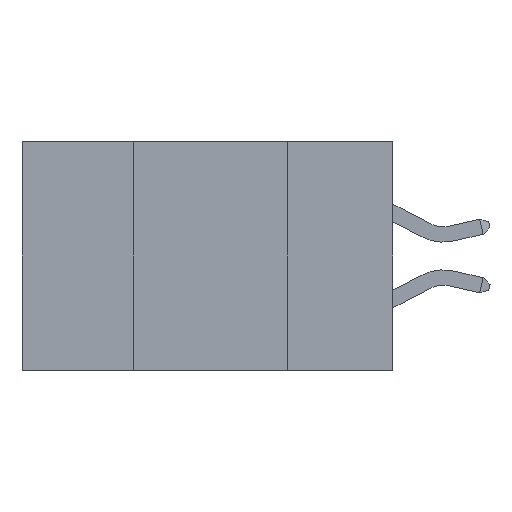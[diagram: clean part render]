
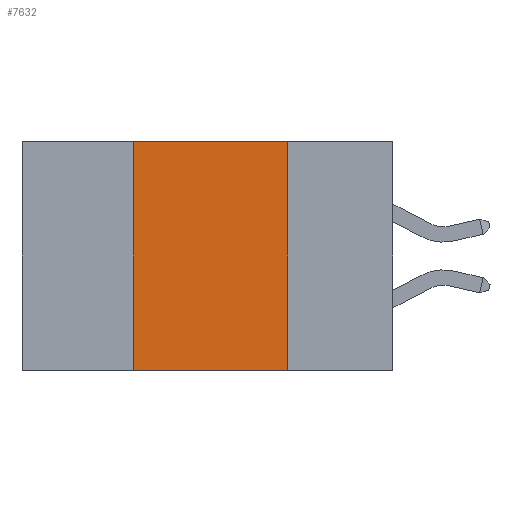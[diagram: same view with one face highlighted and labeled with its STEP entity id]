
A CAD part, left-side view. The second image highlights one B-rep face of the part: STEP entity #7632.
In plain terms, the highlighted planar face has unit normal (-1, 0, 0).
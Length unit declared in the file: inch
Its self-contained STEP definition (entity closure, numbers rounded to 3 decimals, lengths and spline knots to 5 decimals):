
#24 = EDGE_CURVE ( 'NONE', #8611, #7812, #4226, .T. ) ;
#642 = DIRECTION ( 'NONE',  ( 1., 0., 0. ) ) ;
#860 = DIRECTION ( 'NONE',  ( 0., -1., 0. ) ) ;
#1058 = ORIENTED_EDGE ( 'NONE', *, *, #3989, .F. ) ;
#1064 = ORIENTED_EDGE ( 'NONE', *, *, #24, .F. ) ;
#1404 = PLANE ( 'NONE',  #4355 ) ;
#1653 = CARTESIAN_POINT ( 'NONE',  ( 0., 0.17, 0. ) ) ;
#1796 = LINE ( 'NONE', #3952, #2019 ) ;
#1858 = LINE ( 'NONE', #4236, #2079 ) ;
#2019 = VECTOR ( 'NONE', #2530, 39.37008 ) ;
#2022 = DIRECTION ( 'NONE',  ( 0., 0., -1. ) ) ;
#2079 = VECTOR ( 'NONE', #2022, 39.37008 ) ;
#2214 = VECTOR ( 'NONE', #5422, 39.37008 ) ;
#2347 = CARTESIAN_POINT ( 'NONE',  ( 0., 0.6, -0.37 ) ) ;
#2530 = DIRECTION ( 'NONE',  ( 0., -1., 0. ) ) ;
#3100 = FACE_OUTER_BOUND ( 'NONE', #8077, .T. ) ;
#3587 = VERTEX_POINT ( 'NONE', #8003 ) ;
#3935 = EDGE_CURVE ( 'NONE', #8611, #3587, #5152, .T. ) ;
#3952 = CARTESIAN_POINT ( 'NONE',  ( 0., 0.6, 0. ) ) ;
#3989 = EDGE_CURVE ( 'NONE', #7812, #6988, #1796, .T. ) ;
#4226 = LINE ( 'NONE', #8177, #2214 ) ;
#4236 = CARTESIAN_POINT ( 'NONE',  ( 0., 0.17, 0. ) ) ;
#4355 = AXIS2_PLACEMENT_3D ( 'NONE', #8483, #642, #5683 ) ;
#5152 = LINE ( 'NONE', #2347, #7651 ) ;
#5422 = DIRECTION ( 'NONE',  ( 0., 0., 1. ) ) ;
#5683 = DIRECTION ( 'NONE',  ( 0., 0., -1. ) ) ;
#6988 = VERTEX_POINT ( 'NONE', #1653 ) ;
#7632 = ADVANCED_FACE ( 'NONE', ( #3100 ), #1404, .F. ) ;
#7651 = VECTOR ( 'NONE', #860, 39.37008 ) ;
#7812 = VERTEX_POINT ( 'NONE', #7968 ) ;
#7908 = ORIENTED_EDGE ( 'NONE', *, *, #7946, .F. ) ;
#7946 = EDGE_CURVE ( 'NONE', #6988, #3587, #1858, .T. ) ;
#7965 = CARTESIAN_POINT ( 'NONE',  ( 0., 0.42, -0.37 ) ) ;
#7968 = CARTESIAN_POINT ( 'NONE',  ( 0., 0.42, 0. ) ) ;
#8003 = CARTESIAN_POINT ( 'NONE',  ( 0., 0.17, -0.37 ) ) ;
#8077 = EDGE_LOOP ( 'NONE', ( #7908, #1058, #1064, #8278 ) ) ;
#8177 = CARTESIAN_POINT ( 'NONE',  ( 0., 0.42, 0. ) ) ;
#8278 = ORIENTED_EDGE ( 'NONE', *, *, #3935, .T. ) ;
#8483 = CARTESIAN_POINT ( 'NONE',  ( 0., 0.6, 0. ) ) ;
#8611 = VERTEX_POINT ( 'NONE', #7965 ) ;
